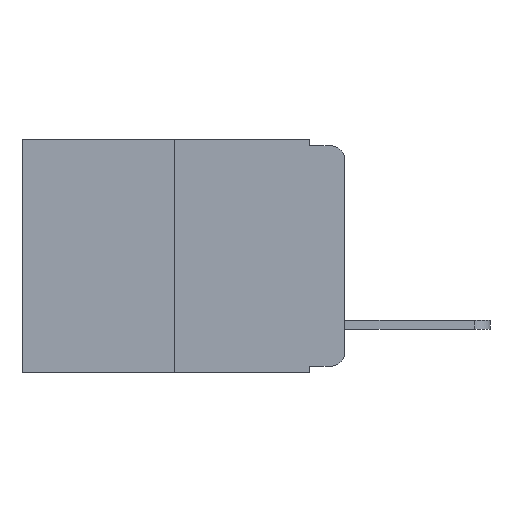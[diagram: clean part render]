
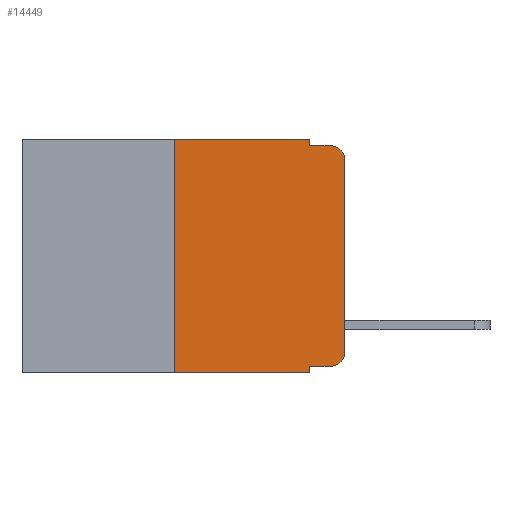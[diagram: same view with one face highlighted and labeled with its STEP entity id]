
A CAD part, left-side view. The second image highlights one B-rep face of the part: STEP entity #14449.
In plain terms, the highlighted planar face has unit normal (-1, 0, 0).
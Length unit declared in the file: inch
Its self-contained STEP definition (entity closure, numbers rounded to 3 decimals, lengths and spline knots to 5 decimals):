
#269 = ORIENTED_EDGE ( 'NONE', *, *, #8565, .F. ) ;
#450 = LINE ( 'NONE', #2442, #9136 ) ;
#466 = ORIENTED_EDGE ( 'NONE', *, *, #19459, .F. ) ;
#626 = ORIENTED_EDGE ( 'NONE', *, *, #19345, .F. ) ;
#1102 = ORIENTED_EDGE ( 'NONE', *, *, #19425, .F. ) ;
#1147 = DIRECTION ( 'NONE',  ( -1., 0., 0. ) ) ;
#1279 = ORIENTED_EDGE ( 'NONE', *, *, #19485, .F. ) ;
#1312 = VERTEX_POINT ( 'NONE', #12058 ) ;
#1352 = AXIS2_PLACEMENT_3D ( 'NONE', #11974, #1147, #13622 ) ;
#1669 = CARTESIAN_POINT ( 'NONE',  ( 0., 0.051, -0.343 ) ) ;
#1924 = DIRECTION ( 'NONE',  ( 0., 0., 1. ) ) ;
#2442 = CARTESIAN_POINT ( 'NONE',  ( 0., 0.25, 0. ) ) ;
#2520 = DIRECTION ( 'NONE',  ( 0., 0., -1. ) ) ;
#3443 = CARTESIAN_POINT ( 'NONE',  ( 0., 0., -0.03 ) ) ;
#3472 = ORIENTED_EDGE ( 'NONE', *, *, #19247, .T. ) ;
#3590 = ORIENTED_EDGE ( 'NONE', *, *, #19275, .T. ) ;
#4069 = AXIS2_PLACEMENT_3D ( 'NONE', #6734, #10508, #22331 ) ;
#4515 = CARTESIAN_POINT ( 'NONE',  ( 0., 0.051, -0.333 ) ) ;
#4570 = VERTEX_POINT ( 'NONE', #16989 ) ;
#4891 = CARTESIAN_POINT ( 'NONE',  ( 0., 0.051, -0.01 ) ) ;
#4899 = LINE ( 'NONE', #12993, #22666 ) ;
#5547 = VECTOR ( 'NONE', #21913, 39.37008 ) ;
#5618 = DIRECTION ( 'NONE',  ( -1., 0., 0. ) ) ;
#5878 = VERTEX_POINT ( 'NONE', #21141 ) ;
#6734 = CARTESIAN_POINT ( 'NONE',  ( 0., 0.473, 0. ) ) ;
#7254 = ORIENTED_EDGE ( 'NONE', *, *, #12953, .T. ) ;
#7582 = VECTOR ( 'NONE', #16712, 39.37008 ) ;
#8216 = CIRCLE ( 'NONE', #22525, 0.02 ) ;
#8281 = VERTEX_POINT ( 'NONE', #4891 ) ;
#8533 = VECTOR ( 'NONE', #16864, 39.37008 ) ;
#8565 = EDGE_CURVE ( 'NONE', #4570, #10511, #19486, .T. ) ;
#8657 = PLANE ( 'NONE',  #4069 ) ;
#9136 = VECTOR ( 'NONE', #19948, 39.37008 ) ;
#9501 = DIRECTION ( 'NONE',  ( 0., -1., 0. ) ) ;
#9746 = LINE ( 'NONE', #4515, #8533 ) ;
#10474 = VERTEX_POINT ( 'NONE', #1669 ) ;
#10508 = DIRECTION ( 'NONE',  ( 1., 0., 0. ) ) ;
#10511 = VERTEX_POINT ( 'NONE', #17281 ) ;
#10825 = LINE ( 'NONE', #21429, #15408 ) ;
#10968 = EDGE_LOOP ( 'NONE', ( #3472, #3590, #626, #1102, #269, #466, #7254, #1279, #14270, #14082 ) ) ;
#11480 = CARTESIAN_POINT ( 'NONE',  ( 0., 0.051, 0. ) ) ;
#11853 = FACE_OUTER_BOUND ( 'NONE', #10968, .T. ) ;
#11974 = CARTESIAN_POINT ( 'NONE',  ( 0., 0.02, -0.313 ) ) ;
#12058 = CARTESIAN_POINT ( 'NONE',  ( 0., 0.02, -0.333 ) ) ;
#12369 = VECTOR ( 'NONE', #1924, 39.37008 ) ;
#12639 = VERTEX_POINT ( 'NONE', #16289 ) ;
#12953 = EDGE_CURVE ( 'NONE', #12639, #10474, #21393, .T. ) ;
#12993 = CARTESIAN_POINT ( 'NONE',  ( 0., 0.051, 0. ) ) ;
#13273 = VERTEX_POINT ( 'NONE', #3443 ) ;
#13622 = DIRECTION ( 'NONE',  ( 0., 0., -1. ) ) ;
#14082 = ORIENTED_EDGE ( 'NONE', *, *, #19701, .T. ) ;
#14123 = CIRCLE ( 'NONE', #1352, 0.02 ) ;
#14270 = ORIENTED_EDGE ( 'NONE', *, *, #19554, .T. ) ;
#14449 = ADVANCED_FACE ( 'NONE', ( #11853 ), #8657, .F. ) ;
#14537 = VERTEX_POINT ( 'NONE', #17669 ) ;
#14845 = DIRECTION ( 'NONE',  ( 0., 0., -1. ) ) ;
#14923 = CARTESIAN_POINT ( 'NONE',  ( 0., 0.473, -0.343 ) ) ;
#15408 = VECTOR ( 'NONE', #9501, 39.37008 ) ;
#16272 = CARTESIAN_POINT ( 'NONE',  ( 0., 0.02, -0.03 ) ) ;
#16289 = CARTESIAN_POINT ( 'NONE',  ( 0., 0.25, -0.343 ) ) ;
#16712 = DIRECTION ( 'NONE',  ( 0., -1., 0. ) ) ;
#16864 = DIRECTION ( 'NONE',  ( 0., -1., 0. ) ) ;
#16989 = CARTESIAN_POINT ( 'NONE',  ( 0., 0.25, 0. ) ) ;
#17281 = CARTESIAN_POINT ( 'NONE',  ( 0., 0.051, 0. ) ) ;
#17588 = CARTESIAN_POINT ( 'NONE',  ( 0., 0.051, -0.333 ) ) ;
#17669 = CARTESIAN_POINT ( 'NONE',  ( 0., 0.02, -0.01 ) ) ;
#17826 = VECTOR ( 'NONE', #2520, 39.37008 ) ;
#17954 = DIRECTION ( 'NONE',  ( 0., 0., -1. ) ) ;
#18097 = LINE ( 'NONE', #22720, #12369 ) ;
#19247 = EDGE_CURVE ( 'NONE', #5878, #13273, #18097, .T. ) ;
#19275 = EDGE_CURVE ( 'NONE', #13273, #14537, #8216, .T. ) ;
#19345 = EDGE_CURVE ( 'NONE', #8281, #14537, #10825, .T. ) ;
#19425 = EDGE_CURVE ( 'NONE', #10511, #8281, #4899, .T. ) ;
#19459 = EDGE_CURVE ( 'NONE', #12639, #4570, #450, .T. ) ;
#19485 = EDGE_CURVE ( 'NONE', #19849, #10474, #22198, .T. ) ;
#19486 = LINE ( 'NONE', #21839, #5547 ) ;
#19554 = EDGE_CURVE ( 'NONE', #19849, #1312, #9746, .T. ) ;
#19701 = EDGE_CURVE ( 'NONE', #1312, #5878, #14123, .T. ) ;
#19849 = VERTEX_POINT ( 'NONE', #17588 ) ;
#19948 = DIRECTION ( 'NONE',  ( 0., 0., 1. ) ) ;
#21141 = CARTESIAN_POINT ( 'NONE',  ( 0., 0., -0.313 ) ) ;
#21393 = LINE ( 'NONE', #14923, #7582 ) ;
#21429 = CARTESIAN_POINT ( 'NONE',  ( 0., 0.051, -0.01 ) ) ;
#21839 = CARTESIAN_POINT ( 'NONE',  ( 0., 0.473, 0. ) ) ;
#21913 = DIRECTION ( 'NONE',  ( 0., -1., 0. ) ) ;
#22198 = LINE ( 'NONE', #11480, #17826 ) ;
#22331 = DIRECTION ( 'NONE',  ( 0., 0., -1. ) ) ;
#22525 = AXIS2_PLACEMENT_3D ( 'NONE', #16272, #5618, #17954 ) ;
#22666 = VECTOR ( 'NONE', #14845, 39.37008 ) ;
#22720 = CARTESIAN_POINT ( 'NONE',  ( 0., 0., 0. ) ) ;
